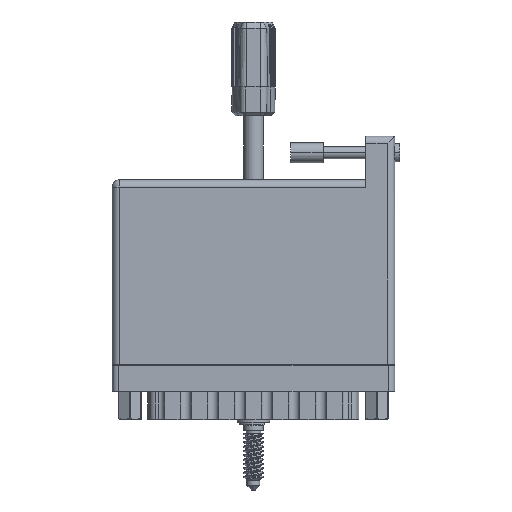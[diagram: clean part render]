
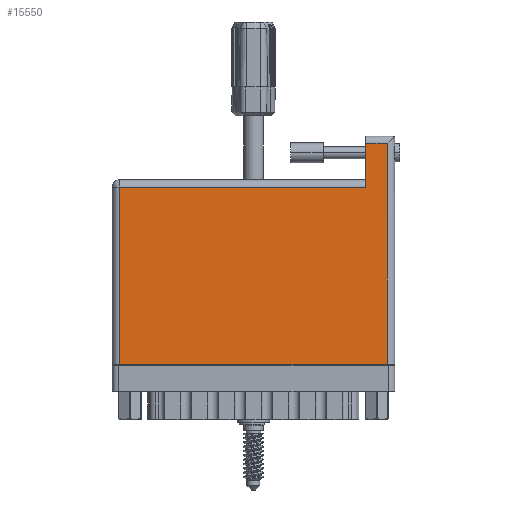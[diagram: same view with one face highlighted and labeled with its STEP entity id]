
A CAD part, front view. The second image highlights one B-rep face of the part: STEP entity #15550.
In plain terms, the highlighted face is planar.
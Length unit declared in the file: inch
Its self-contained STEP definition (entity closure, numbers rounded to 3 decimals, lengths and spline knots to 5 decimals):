
#1220 = LINE ( 'NONE', #49584, #73176 ) ;
#2477 = VECTOR ( 'NONE', #43735, 39.37008 ) ;
#5371 = CARTESIAN_POINT ( 'NONE',  ( 2.438, 2.125, 0. ) ) ;
#9558 = EDGE_CURVE ( 'NONE', #89106, #90597, #80368, .T. ) ;
#9773 = FACE_OUTER_BOUND ( 'NONE', #48830, .T. ) ;
#13564 = CARTESIAN_POINT ( 'NONE',  ( 2.438, 2.195, 0. ) ) ;
#15090 = ORIENTED_EDGE ( 'NONE', *, *, #26907, .T. ) ;
#15550 = ADVANCED_FACE ( 'NONE', ( #9773 ), #60314, .F. ) ;
#18977 = LINE ( 'NONE', #38376, #93231 ) ;
#21558 = VERTEX_POINT ( 'NONE', #88007 ) ;
#22743 = ORIENTED_EDGE ( 'NONE', *, *, #31527, .T. ) ;
#26096 = LINE ( 'NONE', #64718, #2477 ) ;
#26621 = CARTESIAN_POINT ( 'NONE',  ( 2.648, 2.125, 0. ) ) ;
#26907 = EDGE_CURVE ( 'NONE', #67681, #32874, #34417, .T. ) ;
#27909 = DIRECTION ( 'NONE',  ( -1., 0., 0. ) ) ;
#31527 = EDGE_CURVE ( 'NONE', #53047, #89106, #18977, .T. ) ;
#32874 = VERTEX_POINT ( 'NONE', #49701 ) ;
#34417 = LINE ( 'NONE', #92799, #58015 ) ;
#37583 = VECTOR ( 'NONE', #92182, 39.37008 ) ;
#38180 = ORIENTED_EDGE ( 'NONE', *, *, #49160, .T. ) ;
#38376 = CARTESIAN_POINT ( 'NONE',  ( 0., 2.125, 0. ) ) ;
#38526 = ORIENTED_EDGE ( 'NONE', *, *, #67509, .T. ) ;
#38990 = DIRECTION ( 'NONE',  ( -1., 0., 0. ) ) ;
#39931 = DIRECTION ( 'NONE',  ( 0., 0., -1. ) ) ;
#42715 = CARTESIAN_POINT ( 'NONE',  ( 2.438, 1.705, 0. ) ) ;
#43152 = ORIENTED_EDGE ( 'NONE', *, *, #77084, .T. ) ;
#43735 = DIRECTION ( 'NONE',  ( 0., 1., 0. ) ) ;
#48830 = EDGE_LOOP ( 'NONE', ( #38180, #15090, #43152, #38526, #22743, #72733 ) ) ;
#49160 = EDGE_CURVE ( 'NONE', #90597, #67681, #1220, .T. ) ;
#49422 = CARTESIAN_POINT ( 'NONE',  ( 0., 0., 0. ) ) ;
#49584 = CARTESIAN_POINT ( 'NONE',  ( 0., 1.705, 0. ) ) ;
#49701 = CARTESIAN_POINT ( 'NONE',  ( 0.07, 0., 0. ) ) ;
#50956 = DIRECTION ( 'NONE',  ( 0., -1., 0. ) ) ;
#53047 = VERTEX_POINT ( 'NONE', #26621 ) ;
#56716 = AXIS2_PLACEMENT_3D ( 'NONE', #90214, #39931, #38990 ) ;
#57197 = CARTESIAN_POINT ( 'NONE',  ( 0.07, 1.705, 0. ) ) ;
#58015 = VECTOR ( 'NONE', #50956, 39.37008 ) ;
#60314 = PLANE ( 'NONE',  #56716 ) ;
#64718 = CARTESIAN_POINT ( 'NONE',  ( 2.648, 2.195, 0. ) ) ;
#67509 = EDGE_CURVE ( 'NONE', #21558, #53047, #26096, .T. ) ;
#67681 = VERTEX_POINT ( 'NONE', #57197 ) ;
#72733 = ORIENTED_EDGE ( 'NONE', *, *, #9558, .T. ) ;
#73176 = VECTOR ( 'NONE', #27909, 39.37008 ) ;
#74767 = VECTOR ( 'NONE', #78309, 39.37008 ) ;
#75784 = LINE ( 'NONE', #49422, #37583 ) ;
#77084 = EDGE_CURVE ( 'NONE', #32874, #21558, #75784, .T. ) ;
#78309 = DIRECTION ( 'NONE',  ( 0., -1., 0. ) ) ;
#80368 = LINE ( 'NONE', #13564, #74767 ) ;
#81738 = DIRECTION ( 'NONE',  ( -1., 0., 0. ) ) ;
#88007 = CARTESIAN_POINT ( 'NONE',  ( 2.648, 0., 0. ) ) ;
#89106 = VERTEX_POINT ( 'NONE', #5371 ) ;
#90214 = CARTESIAN_POINT ( 'NONE',  ( 0., 1.775, 0. ) ) ;
#90597 = VERTEX_POINT ( 'NONE', #42715 ) ;
#92182 = DIRECTION ( 'NONE',  ( 1., 0., 0. ) ) ;
#92799 = CARTESIAN_POINT ( 'NONE',  ( 0.07, 0., 0. ) ) ;
#93231 = VECTOR ( 'NONE', #81738, 39.37008 ) ;
